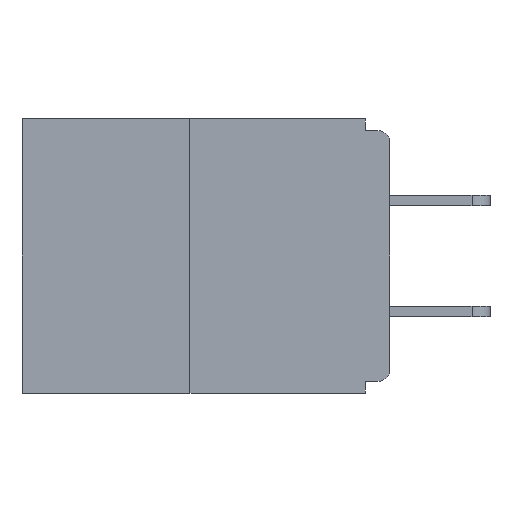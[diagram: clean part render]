
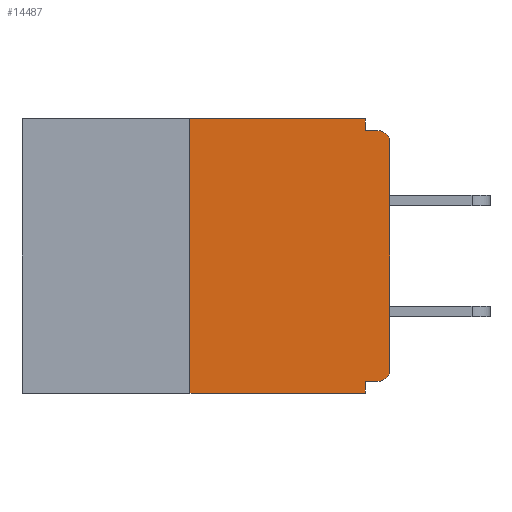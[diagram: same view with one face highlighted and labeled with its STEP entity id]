
A CAD part, left-side view. The second image highlights one B-rep face of the part: STEP entity #14487.
In plain terms, the highlighted planar face has unit normal (-1, 0, 0).
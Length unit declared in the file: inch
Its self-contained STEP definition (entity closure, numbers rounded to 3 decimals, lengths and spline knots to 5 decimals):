
#538 = LINE ( 'NONE', #23916, #5216 ) ;
#691 = CARTESIAN_POINT ( 'NONE',  ( 0., 0.015, -0.015 ) ) ;
#2246 = CARTESIAN_POINT ( 'NONE',  ( 0., 0.46, 0. ) ) ;
#2522 = EDGE_CURVE ( 'NONE', #17463, #17364, #24477, .T. ) ;
#2569 = LINE ( 'NONE', #29154, #13811 ) ;
#2585 = DIRECTION ( 'NONE',  ( 0., 0., 1. ) ) ;
#2763 = EDGE_CURVE ( 'NONE', #7275, #19416, #9520, .T. ) ;
#4159 = LINE ( 'NONE', #2246, #24843 ) ;
#4221 = VECTOR ( 'NONE', #14332, 39.37008 ) ;
#4270 = CARTESIAN_POINT ( 'NONE',  ( 0., 0.25, 0. ) ) ;
#4784 = ORIENTED_EDGE ( 'NONE', *, *, #2522, .F. ) ;
#4980 = CARTESIAN_POINT ( 'NONE',  ( 0., 0.031, -0.343 ) ) ;
#5216 = VECTOR ( 'NONE', #7678, 39.37008 ) ;
#5597 = CARTESIAN_POINT ( 'NONE',  ( 0., 0.015, -0.328 ) ) ;
#5998 = ORIENTED_EDGE ( 'NONE', *, *, #22254, .F. ) ;
#6937 = CARTESIAN_POINT ( 'NONE',  ( 0., 0.015, -0.03 ) ) ;
#7275 = VERTEX_POINT ( 'NONE', #21918 ) ;
#7488 = CARTESIAN_POINT ( 'NONE',  ( 0., 0.031, -0.343 ) ) ;
#7564 = CARTESIAN_POINT ( 'NONE',  ( 0., 0.031, 0. ) ) ;
#7629 = EDGE_LOOP ( 'NONE', ( #29894, #5998, #16724, #4784, #26232, #10087, #20298, #13178, #14553, #13619 ) ) ;
#7678 = DIRECTION ( 'NONE',  ( 0., 1., 0. ) ) ;
#9029 = CARTESIAN_POINT ( 'NONE',  ( 0., 0.46, 0. ) ) ;
#9469 = AXIS2_PLACEMENT_3D ( 'NONE', #18563, #9554, #20876 ) ;
#9516 = VERTEX_POINT ( 'NONE', #20369 ) ;
#9520 = CIRCLE ( 'NONE', #16407, 0.015 ) ;
#9554 = DIRECTION ( 'NONE',  ( -1., 0., 0. ) ) ;
#9631 = DIRECTION ( 'NONE',  ( 0., 0., 1. ) ) ;
#9767 = EDGE_CURVE ( 'NONE', #9516, #7275, #20584, .T. ) ;
#10087 = ORIENTED_EDGE ( 'NONE', *, *, #28550, .T. ) ;
#10953 = AXIS2_PLACEMENT_3D ( 'NONE', #9029, #15867, #25330 ) ;
#11079 = VECTOR ( 'NONE', #9631, 39.37008 ) ;
#11968 = CARTESIAN_POINT ( 'NONE',  ( 0., 0., -0.015 ) ) ;
#13092 = CARTESIAN_POINT ( 'NONE',  ( 0., 0.031, -0.015 ) ) ;
#13178 = ORIENTED_EDGE ( 'NONE', *, *, #2763, .T. ) ;
#13297 = LINE ( 'NONE', #18935, #11079 ) ;
#13619 = ORIENTED_EDGE ( 'NONE', *, *, #18287, .F. ) ;
#13811 = VECTOR ( 'NONE', #24872, 39.37008 ) ;
#13887 = VERTEX_POINT ( 'NONE', #23560 ) ;
#14332 = DIRECTION ( 'NONE',  ( 0., -1., 0. ) ) ;
#14398 = VECTOR ( 'NONE', #2585, 39.37008 ) ;
#14471 = EDGE_CURVE ( 'NONE', #13887, #17364, #2569, .T. ) ;
#14487 = ADVANCED_FACE ( 'NONE', ( #21064 ), #25625, .F. ) ;
#14553 = ORIENTED_EDGE ( 'NONE', *, *, #23009, .F. ) ;
#15867 = DIRECTION ( 'NONE',  ( 1., 0., 0. ) ) ;
#16299 = DIRECTION ( 'NONE',  ( 0., 0., -1. ) ) ;
#16345 = VERTEX_POINT ( 'NONE', #13092 ) ;
#16407 = AXIS2_PLACEMENT_3D ( 'NONE', #6937, #27943, #16299 ) ;
#16724 = ORIENTED_EDGE ( 'NONE', *, *, #14471, .T. ) ;
#17083 = EDGE_CURVE ( 'NONE', #23795, #17463, #538, .T. ) ;
#17364 = VERTEX_POINT ( 'NONE', #4980 ) ;
#17463 = VERTEX_POINT ( 'NONE', #28569 ) ;
#18287 = EDGE_CURVE ( 'NONE', #21830, #16345, #21484, .T. ) ;
#18322 = VECTOR ( 'NONE', #18704, 39.37008 ) ;
#18563 = CARTESIAN_POINT ( 'NONE',  ( 0., 0.015, -0.313 ) ) ;
#18621 = VECTOR ( 'NONE', #19439, 39.37008 ) ;
#18704 = DIRECTION ( 'NONE',  ( 0., 0., -1. ) ) ;
#18935 = CARTESIAN_POINT ( 'NONE',  ( 0., 0.25, 0. ) ) ;
#19416 = VERTEX_POINT ( 'NONE', #691 ) ;
#19439 = DIRECTION ( 'NONE',  ( 0., 0., -1. ) ) ;
#19643 = CARTESIAN_POINT ( 'NONE',  ( 0., 0.031, 0. ) ) ;
#20298 = ORIENTED_EDGE ( 'NONE', *, *, #9767, .T. ) ;
#20369 = CARTESIAN_POINT ( 'NONE',  ( 0., 0., -0.313 ) ) ;
#20584 = LINE ( 'NONE', #20931, #14398 ) ;
#20680 = DIRECTION ( 'NONE',  ( 0., -1., 0. ) ) ;
#20876 = DIRECTION ( 'NONE',  ( 0., 0., -1. ) ) ;
#20931 = CARTESIAN_POINT ( 'NONE',  ( 0., 0., 0. ) ) ;
#21064 = FACE_OUTER_BOUND ( 'NONE', #7629, .T. ) ;
#21484 = LINE ( 'NONE', #19643, #18621 ) ;
#21830 = VERTEX_POINT ( 'NONE', #7564 ) ;
#21918 = CARTESIAN_POINT ( 'NONE',  ( 0., 0., -0.03 ) ) ;
#22254 = EDGE_CURVE ( 'NONE', #13887, #28560, #13297, .T. ) ;
#23009 = EDGE_CURVE ( 'NONE', #16345, #19416, #27781, .T. ) ;
#23560 = CARTESIAN_POINT ( 'NONE',  ( 0., 0.25, -0.343 ) ) ;
#23795 = VERTEX_POINT ( 'NONE', #5597 ) ;
#23916 = CARTESIAN_POINT ( 'NONE',  ( 0., 0., -0.328 ) ) ;
#24477 = LINE ( 'NONE', #7488, #18322 ) ;
#24843 = VECTOR ( 'NONE', #20680, 39.37008 ) ;
#24872 = DIRECTION ( 'NONE',  ( 0., -1., 0. ) ) ;
#25330 = DIRECTION ( 'NONE',  ( 0., 0., -1. ) ) ;
#25596 = CIRCLE ( 'NONE', #9469, 0.015 ) ;
#25625 = PLANE ( 'NONE',  #10953 ) ;
#26232 = ORIENTED_EDGE ( 'NONE', *, *, #17083, .F. ) ;
#27781 = LINE ( 'NONE', #11968, #4221 ) ;
#27943 = DIRECTION ( 'NONE',  ( -1., 0., 0. ) ) ;
#28504 = EDGE_CURVE ( 'NONE', #28560, #21830, #4159, .T. ) ;
#28550 = EDGE_CURVE ( 'NONE', #23795, #9516, #25596, .T. ) ;
#28560 = VERTEX_POINT ( 'NONE', #4270 ) ;
#28569 = CARTESIAN_POINT ( 'NONE',  ( 0., 0.031, -0.328 ) ) ;
#29154 = CARTESIAN_POINT ( 'NONE',  ( 0., 0.46, -0.343 ) ) ;
#29894 = ORIENTED_EDGE ( 'NONE', *, *, #28504, .F. ) ;
